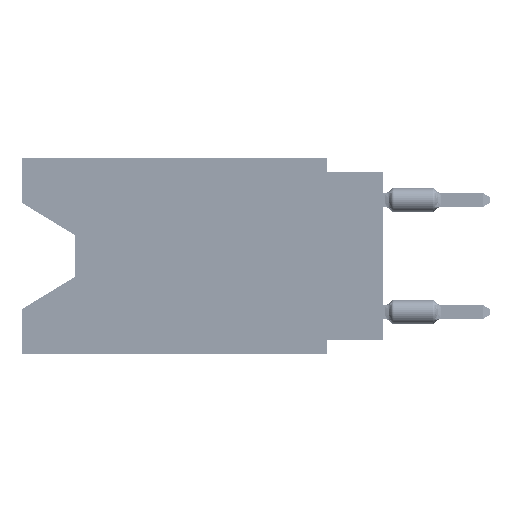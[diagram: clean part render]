
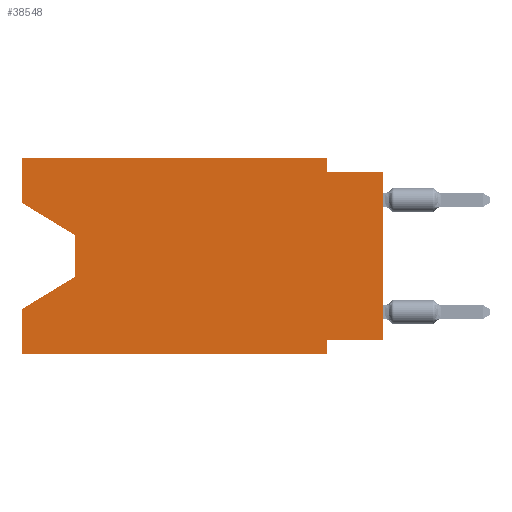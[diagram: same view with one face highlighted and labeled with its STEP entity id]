
A CAD part, left-side view. The second image highlights one B-rep face of the part: STEP entity #38548.
In plain terms, the highlighted planar face has unit normal (-1, 0, 0).
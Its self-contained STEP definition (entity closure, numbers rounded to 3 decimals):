
#2062 = VERTEX_POINT ( 'NONE', #18739 ) ;
#2182 = CARTESIAN_POINT ( 'NONE',  ( 0., 16.383, 0. ) ) ;
#2817 = DIRECTION ( 'NONE',  ( 0., 0., 1. ) ) ;
#4089 = CARTESIAN_POINT ( 'NONE',  ( 0., 16.383, 0. ) ) ;
#4230 = EDGE_CURVE ( 'NONE', #45944, #20532, #26573, .T. ) ;
#4334 = VECTOR ( 'NONE', #21229, 1000. ) ;
#5019 = CARTESIAN_POINT ( 'NONE',  ( 0., 16.383, -6.852 ) ) ;
#5619 = CARTESIAN_POINT ( 'NONE',  ( 0., 2.54, -0.635 ) ) ;
#5630 = VECTOR ( 'NONE', #26132, 1000. ) ;
#7852 = EDGE_CURVE ( 'NONE', #47177, #8714, #47869, .T. ) ;
#8408 = VECTOR ( 'NONE', #11387, 1000. ) ;
#8714 = VERTEX_POINT ( 'NONE', #5019 ) ;
#9667 = LINE ( 'NONE', #53055, #36620 ) ;
#10044 = VERTEX_POINT ( 'NONE', #59280 ) ;
#11122 = VECTOR ( 'NONE', #54387, 1000. ) ;
#11249 = VECTOR ( 'NONE', #33204, 1000. ) ;
#11387 = DIRECTION ( 'NONE',  ( 0., 0., -1. ) ) ;
#11833 = VERTEX_POINT ( 'NONE', #52298 ) ;
#12024 = DIRECTION ( 'NONE',  ( 0., 0., -1. ) ) ;
#13754 = ORIENTED_EDGE ( 'NONE', *, *, #56316, .F. ) ;
#14139 = CARTESIAN_POINT ( 'NONE',  ( 0., 0., -0.635 ) ) ;
#14892 = CARTESIAN_POINT ( 'NONE',  ( 0., 0., -0.635 ) ) ;
#15581 = EDGE_CURVE ( 'NONE', #43467, #2062, #49706, .T. ) ;
#15929 = LINE ( 'NONE', #2182, #4334 ) ;
#16673 = LINE ( 'NONE', #30450, #8408 ) ;
#18292 = LINE ( 'NONE', #46119, #56273 ) ;
#18697 = EDGE_CURVE ( 'NONE', #47003, #43467, #9667, .T. ) ;
#18739 = CARTESIAN_POINT ( 'NONE',  ( 0., 13.97, -5.385 ) ) ;
#18840 = CARTESIAN_POINT ( 'NONE',  ( 0., 16.383, 0. ) ) ;
#19587 = ORIENTED_EDGE ( 'NONE', *, *, #7852, .F. ) ;
#20532 = VERTEX_POINT ( 'NONE', #14892 ) ;
#20568 = ORIENTED_EDGE ( 'NONE', *, *, #18697, .T. ) ;
#21229 = DIRECTION ( 'NONE',  ( 0., -1., 0. ) ) ;
#21440 = ORIENTED_EDGE ( 'NONE', *, *, #15581, .T. ) ;
#22522 = DIRECTION ( 'NONE',  ( 0., -0.855, -0.519 ) ) ;
#23507 = EDGE_CURVE ( 'NONE', #24179, #20532, #50173, .T. ) ;
#23742 = CARTESIAN_POINT ( 'NONE',  ( 0., 2.54, 0. ) ) ;
#24179 = VERTEX_POINT ( 'NONE', #5619 ) ;
#24888 = CARTESIAN_POINT ( 'NONE',  ( 0., 16.383, -2.038 ) ) ;
#26006 = CARTESIAN_POINT ( 'NONE',  ( 0., 13.97, -3.505 ) ) ;
#26097 = CARTESIAN_POINT ( 'NONE',  ( 0., 2.54, 0. ) ) ;
#26132 = DIRECTION ( 'NONE',  ( 0., -1., 0. ) ) ;
#26410 = DIRECTION ( 'NONE',  ( 0., 1., 0. ) ) ;
#26573 = LINE ( 'NONE', #45610, #31863 ) ;
#26708 = ORIENTED_EDGE ( 'NONE', *, *, #35967, .F. ) ;
#28996 = EDGE_LOOP ( 'NONE', ( #20568, #21440, #51273, #19587, #39816, #13754, #45286, #48608, #48466, #26708, #38277, #32570 ) ) ;
#30450 = CARTESIAN_POINT ( 'NONE',  ( 0., 2.54, -8.89 ) ) ;
#30778 = LINE ( 'NONE', #26097, #54322 ) ;
#31863 = VECTOR ( 'NONE', #2817, 1000. ) ;
#32511 = EDGE_CURVE ( 'NONE', #2062, #8714, #40017, .T. ) ;
#32570 = ORIENTED_EDGE ( 'NONE', *, *, #44581, .F. ) ;
#32723 = VERTEX_POINT ( 'NONE', #23742 ) ;
#33204 = DIRECTION ( 'NONE',  ( 0., 0., 1. ) ) ;
#34319 = PLANE ( 'NONE',  #61787 ) ;
#35062 = EDGE_CURVE ( 'NONE', #59910, #32723, #15929, .T. ) ;
#35754 = CARTESIAN_POINT ( 'NONE',  ( 0., 0., -8.255 ) ) ;
#35967 = EDGE_CURVE ( 'NONE', #32723, #24179, #30778, .T. ) ;
#36409 = CARTESIAN_POINT ( 'NONE',  ( 0., 16.383, -8.89 ) ) ;
#36620 = VECTOR ( 'NONE', #22522, 1000. ) ;
#38277 = ORIENTED_EDGE ( 'NONE', *, *, #35062, .F. ) ;
#38548 = ADVANCED_FACE ( 'NONE', ( #38685 ), #34319, .F. ) ;
#38685 = FACE_OUTER_BOUND ( 'NONE', #28996, .T. ) ;
#39816 = ORIENTED_EDGE ( 'NONE', *, *, #47097, .T. ) ;
#40017 = LINE ( 'NONE', #60020, #11122 ) ;
#40344 = DIRECTION ( 'NONE',  ( 0., 0., -1. ) ) ;
#40439 = LINE ( 'NONE', #35754, #52820 ) ;
#43069 = CARTESIAN_POINT ( 'NONE',  ( 0., 16.383, 0. ) ) ;
#43467 = VERTEX_POINT ( 'NONE', #53245 ) ;
#43672 = DIRECTION ( 'NONE',  ( 1., 0., 0. ) ) ;
#44581 = EDGE_CURVE ( 'NONE', #47003, #59910, #18292, .T. ) ;
#45286 = ORIENTED_EDGE ( 'NONE', *, *, #61006, .F. ) ;
#45610 = CARTESIAN_POINT ( 'NONE',  ( 0., 0., 0. ) ) ;
#45808 = DIRECTION ( 'NONE',  ( 0., -1., 0. ) ) ;
#45944 = VERTEX_POINT ( 'NONE', #54833 ) ;
#46119 = CARTESIAN_POINT ( 'NONE',  ( 0., 16.383, 0. ) ) ;
#47003 = VERTEX_POINT ( 'NONE', #24888 ) ;
#47097 = EDGE_CURVE ( 'NONE', #47177, #11833, #54844, .T. ) ;
#47177 = VERTEX_POINT ( 'NONE', #36409 ) ;
#47869 = LINE ( 'NONE', #18840, #11249 ) ;
#48466 = ORIENTED_EDGE ( 'NONE', *, *, #23507, .F. ) ;
#48476 = VECTOR ( 'NONE', #40344, 1000. ) ;
#48608 = ORIENTED_EDGE ( 'NONE', *, *, #4230, .T. ) ;
#49706 = LINE ( 'NONE', #26006, #48476 ) ;
#50173 = LINE ( 'NONE', #14139, #55114 ) ;
#51273 = ORIENTED_EDGE ( 'NONE', *, *, #32511, .T. ) ;
#52298 = CARTESIAN_POINT ( 'NONE',  ( 0., 2.54, -8.89 ) ) ;
#52820 = VECTOR ( 'NONE', #26410, 1000. ) ;
#53055 = CARTESIAN_POINT ( 'NONE',  ( 0., 16.383, -2.038 ) ) ;
#53245 = CARTESIAN_POINT ( 'NONE',  ( 0., 13.97, -3.505 ) ) ;
#53354 = DIRECTION ( 'NONE',  ( 0., 0., -1. ) ) ;
#54322 = VECTOR ( 'NONE', #12024, 1000. ) ;
#54387 = DIRECTION ( 'NONE',  ( 0., 0.855, -0.519 ) ) ;
#54833 = CARTESIAN_POINT ( 'NONE',  ( 0., 0., -8.255 ) ) ;
#54844 = LINE ( 'NONE', #55759, #5630 ) ;
#55114 = VECTOR ( 'NONE', #45808, 1000. ) ;
#55759 = CARTESIAN_POINT ( 'NONE',  ( 0., 16.383, -8.89 ) ) ;
#56273 = VECTOR ( 'NONE', #60201, 1000. ) ;
#56316 = EDGE_CURVE ( 'NONE', #10044, #11833, #16673, .T. ) ;
#59280 = CARTESIAN_POINT ( 'NONE',  ( 0., 2.54, -8.255 ) ) ;
#59910 = VERTEX_POINT ( 'NONE', #4089 ) ;
#60020 = CARTESIAN_POINT ( 'NONE',  ( 0., 13.97, -5.385 ) ) ;
#60201 = DIRECTION ( 'NONE',  ( 0., 0., 1. ) ) ;
#61006 = EDGE_CURVE ( 'NONE', #45944, #10044, #40439, .T. ) ;
#61787 = AXIS2_PLACEMENT_3D ( 'NONE', #43069, #43672, #53354 ) ;
